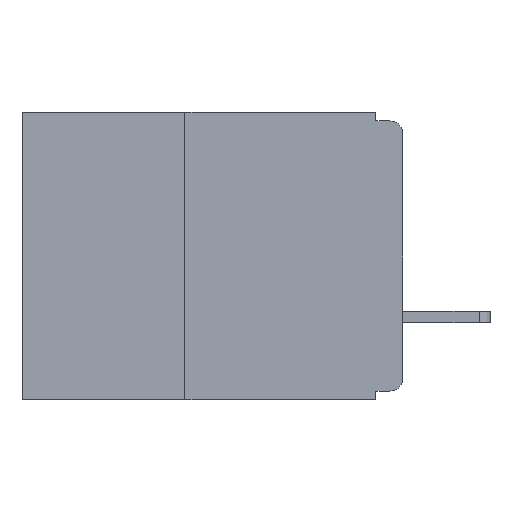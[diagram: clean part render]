
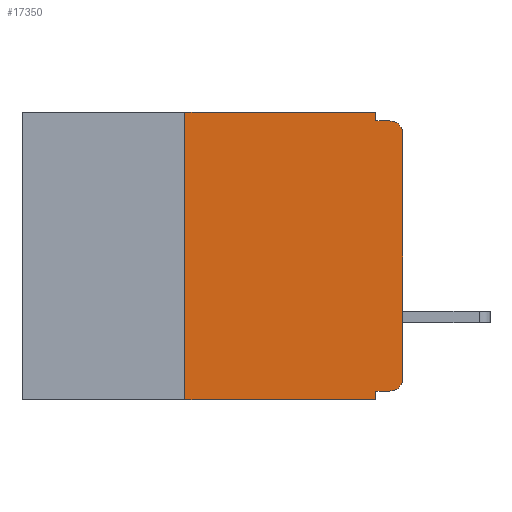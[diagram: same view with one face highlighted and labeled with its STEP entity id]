
A CAD part, left-side view. The second image highlights one B-rep face of the part: STEP entity #17350.
In plain terms, the highlighted planar face has unit normal (-1, 0, 0).
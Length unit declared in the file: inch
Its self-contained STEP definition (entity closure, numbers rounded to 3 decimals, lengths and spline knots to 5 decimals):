
#849 = CARTESIAN_POINT ( 'NONE',  ( 0., 0.031, -0.01 ) ) ;
#1895 = VECTOR ( 'NONE', #2992, 39.37008 ) ;
#2124 = VERTEX_POINT ( 'NONE', #27457 ) ;
#2519 = VECTOR ( 'NONE', #14608, 39.37008 ) ;
#2992 = DIRECTION ( 'NONE',  ( 0., -1., 0. ) ) ;
#3665 = VECTOR ( 'NONE', #11408, 39.37008 ) ;
#3861 = DIRECTION ( 'NONE',  ( 1., 0., 0. ) ) ;
#4419 = CARTESIAN_POINT ( 'NONE',  ( 0., 0.25, -0.33 ) ) ;
#4817 = CARTESIAN_POINT ( 'NONE',  ( 0., 0.015, -0.32 ) ) ;
#5314 = VERTEX_POINT ( 'NONE', #27635 ) ;
#5705 = CARTESIAN_POINT ( 'NONE',  ( 0., 0.015, -0.025 ) ) ;
#5859 = VERTEX_POINT ( 'NONE', #4817 ) ;
#6319 = AXIS2_PLACEMENT_3D ( 'NONE', #28565, #3861, #21262 ) ;
#6597 = DIRECTION ( 'NONE',  ( 0., 1., 0. ) ) ;
#8041 = CARTESIAN_POINT ( 'NONE',  ( 0., 0.437, 0. ) ) ;
#8128 = CARTESIAN_POINT ( 'NONE',  ( 0., 0.031, -0.33 ) ) ;
#8201 = EDGE_LOOP ( 'NONE', ( #16504, #17399, #28635, #29378, #24072, #31866, #21867, #17242, #30654, #9344 ) ) ;
#8225 = DIRECTION ( 'NONE',  ( 0., 0., -1. ) ) ;
#8748 = LINE ( 'NONE', #16541, #27719 ) ;
#8899 = CARTESIAN_POINT ( 'NONE',  ( 0., 0.031, 0. ) ) ;
#9276 = VECTOR ( 'NONE', #19323, 39.37008 ) ;
#9344 = ORIENTED_EDGE ( 'NONE', *, *, #30711, .T. ) ;
#9452 = CARTESIAN_POINT ( 'NONE',  ( 0., 0.437, -0.33 ) ) ;
#9794 = DIRECTION ( 'NONE',  ( -1., 0., 0. ) ) ;
#10650 = EDGE_CURVE ( 'NONE', #13489, #27143, #14914, .T. ) ;
#11235 = CARTESIAN_POINT ( 'NONE',  ( 0., 0., -0.025 ) ) ;
#11408 = DIRECTION ( 'NONE',  ( 0., 0., -1. ) ) ;
#11459 = DIRECTION ( 'NONE',  ( 0., -1., 0. ) ) ;
#11769 = CARTESIAN_POINT ( 'NONE',  ( 0., 0., -0.305 ) ) ;
#12000 = CIRCLE ( 'NONE', #25751, 0.015 ) ;
#12172 = VERTEX_POINT ( 'NONE', #25891 ) ;
#13489 = VERTEX_POINT ( 'NONE', #11769 ) ;
#13792 = EDGE_CURVE ( 'NONE', #2124, #5314, #21775, .T. ) ;
#14608 = DIRECTION ( 'NONE',  ( 0., -1., 0. ) ) ;
#14914 = LINE ( 'NONE', #20481, #27235 ) ;
#15004 = VERTEX_POINT ( 'NONE', #25679 ) ;
#15936 = LINE ( 'NONE', #4419, #9276 ) ;
#16374 = CARTESIAN_POINT ( 'NONE',  ( 0., 0., -0.01 ) ) ;
#16398 = EDGE_CURVE ( 'NONE', #12172, #21412, #22387, .T. ) ;
#16448 = CARTESIAN_POINT ( 'NONE',  ( 0., 0.015, -0.01 ) ) ;
#16504 = ORIENTED_EDGE ( 'NONE', *, *, #10650, .T. ) ;
#16541 = CARTESIAN_POINT ( 'NONE',  ( 0., 0., -0.32 ) ) ;
#17242 = ORIENTED_EDGE ( 'NONE', *, *, #26367, .F. ) ;
#17350 = ADVANCED_FACE ( 'NONE', ( #17728 ), #18774, .F. ) ;
#17362 = EDGE_CURVE ( 'NONE', #5314, #22561, #23472, .T. ) ;
#17399 = ORIENTED_EDGE ( 'NONE', *, *, #31625, .T. ) ;
#17402 = EDGE_CURVE ( 'NONE', #5859, #15004, #8748, .T. ) ;
#17728 = FACE_OUTER_BOUND ( 'NONE', #8201, .T. ) ;
#18774 = PLANE ( 'NONE',  #6319 ) ;
#19323 = DIRECTION ( 'NONE',  ( 0., 0., 1. ) ) ;
#20481 = CARTESIAN_POINT ( 'NONE',  ( 0., 0., 0. ) ) ;
#21262 = DIRECTION ( 'NONE',  ( 0., 0., -1. ) ) ;
#21412 = VERTEX_POINT ( 'NONE', #28206 ) ;
#21775 = LINE ( 'NONE', #8041, #1895 ) ;
#21867 = ORIENTED_EDGE ( 'NONE', *, *, #16398, .T. ) ;
#22387 = LINE ( 'NONE', #9452, #2519 ) ;
#22561 = VERTEX_POINT ( 'NONE', #849 ) ;
#22949 = DIRECTION ( 'NONE',  ( 0., 0., 1. ) ) ;
#23066 = DIRECTION ( 'NONE',  ( -1., 0., 0. ) ) ;
#23147 = EDGE_CURVE ( 'NONE', #22561, #25549, #31570, .T. ) ;
#23472 = LINE ( 'NONE', #8899, #3665 ) ;
#23716 = LINE ( 'NONE', #8128, #29467 ) ;
#24072 = ORIENTED_EDGE ( 'NONE', *, *, #13792, .F. ) ;
#24187 = AXIS2_PLACEMENT_3D ( 'NONE', #24633, #9794, #27100 ) ;
#24633 = CARTESIAN_POINT ( 'NONE',  ( 0., 0.015, -0.305 ) ) ;
#25125 = VECTOR ( 'NONE', #11459, 39.37008 ) ;
#25549 = VERTEX_POINT ( 'NONE', #16448 ) ;
#25679 = CARTESIAN_POINT ( 'NONE',  ( 0., 0.031, -0.32 ) ) ;
#25751 = AXIS2_PLACEMENT_3D ( 'NONE', #5705, #23066, #8225 ) ;
#25891 = CARTESIAN_POINT ( 'NONE',  ( 0., 0.25, -0.33 ) ) ;
#26367 = EDGE_CURVE ( 'NONE', #15004, #21412, #23716, .T. ) ;
#27100 = DIRECTION ( 'NONE',  ( 0., 0., -1. ) ) ;
#27143 = VERTEX_POINT ( 'NONE', #11235 ) ;
#27235 = VECTOR ( 'NONE', #22949, 39.37008 ) ;
#27457 = CARTESIAN_POINT ( 'NONE',  ( 0., 0.25, 0. ) ) ;
#27517 = CIRCLE ( 'NONE', #24187, 0.015 ) ;
#27635 = CARTESIAN_POINT ( 'NONE',  ( 0., 0.031, 0. ) ) ;
#27719 = VECTOR ( 'NONE', #6597, 39.37008 ) ;
#27884 = EDGE_CURVE ( 'NONE', #12172, #2124, #15936, .T. ) ;
#28206 = CARTESIAN_POINT ( 'NONE',  ( 0., 0.031, -0.33 ) ) ;
#28565 = CARTESIAN_POINT ( 'NONE',  ( 0., 0.437, 0. ) ) ;
#28635 = ORIENTED_EDGE ( 'NONE', *, *, #23147, .F. ) ;
#29378 = ORIENTED_EDGE ( 'NONE', *, *, #17362, .F. ) ;
#29467 = VECTOR ( 'NONE', #30358, 39.37008 ) ;
#30358 = DIRECTION ( 'NONE',  ( 0., 0., -1. ) ) ;
#30654 = ORIENTED_EDGE ( 'NONE', *, *, #17402, .F. ) ;
#30711 = EDGE_CURVE ( 'NONE', #5859, #13489, #27517, .T. ) ;
#31570 = LINE ( 'NONE', #16374, #25125 ) ;
#31625 = EDGE_CURVE ( 'NONE', #27143, #25549, #12000, .T. ) ;
#31866 = ORIENTED_EDGE ( 'NONE', *, *, #27884, .F. ) ;
